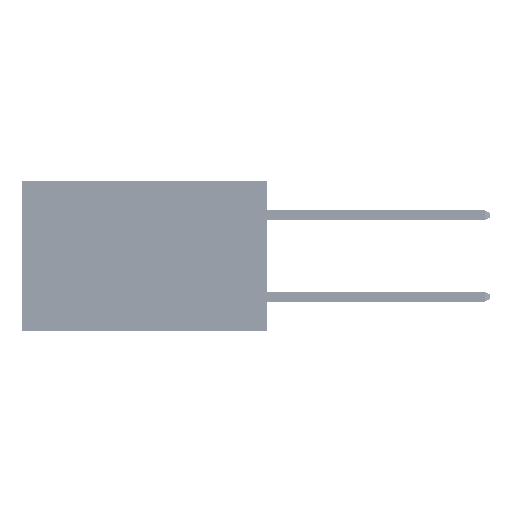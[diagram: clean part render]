
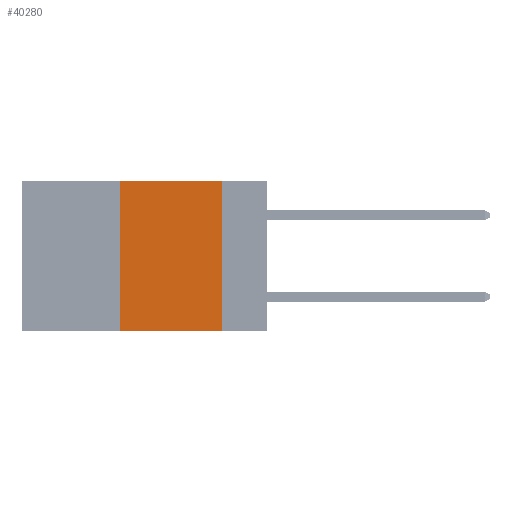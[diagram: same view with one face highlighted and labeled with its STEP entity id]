
A CAD part, left-side view. The second image highlights one B-rep face of the part: STEP entity #40280.
In plain terms, the highlighted planar face has unit normal (-1, 0, 0).
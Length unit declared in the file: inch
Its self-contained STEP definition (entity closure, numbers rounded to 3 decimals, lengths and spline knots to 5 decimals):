
#652 = EDGE_CURVE ( 'NONE', #5444, #50497, #5335, .T. ) ;
#2498 = CARTESIAN_POINT ( 'NONE',  ( 0., 0.11, 0. ) ) ;
#3532 = VECTOR ( 'NONE', #49097, 39.37008 ) ;
#4040 = CARTESIAN_POINT ( 'NONE',  ( 0., 0.36, 0. ) ) ;
#4802 = FACE_OUTER_BOUND ( 'NONE', #23849, .T. ) ;
#4806 = PLANE ( 'NONE',  #24379 ) ;
#5335 = LINE ( 'NONE', #4040, #3532 ) ;
#5444 = VERTEX_POINT ( 'NONE', #21013 ) ;
#6139 = DIRECTION ( 'NONE',  ( 0., -1., 0. ) ) ;
#6668 = LINE ( 'NONE', #2498, #26989 ) ;
#8266 = LINE ( 'NONE', #50133, #28001 ) ;
#8315 = EDGE_CURVE ( 'NONE', #50497, #37248, #40136, .T. ) ;
#9761 = ORIENTED_EDGE ( 'NONE', *, *, #8315, .F. ) ;
#9820 = ORIENTED_EDGE ( 'NONE', *, *, #652, .F. ) ;
#10383 = CARTESIAN_POINT ( 'NONE',  ( 0., 0.6, 0. ) ) ;
#13684 = DIRECTION ( 'NONE',  ( 0., 0., -1. ) ) ;
#18819 = DIRECTION ( 'NONE',  ( 0., 0., -1. ) ) ;
#21013 = CARTESIAN_POINT ( 'NONE',  ( 0., 0.36, -0.37 ) ) ;
#21772 = DIRECTION ( 'NONE',  ( 0., -1., 0. ) ) ;
#21999 = CARTESIAN_POINT ( 'NONE',  ( 0., 0.36, 0. ) ) ;
#23849 = EDGE_LOOP ( 'NONE', ( #24038, #9761, #9820, #44391 ) ) ;
#24038 = ORIENTED_EDGE ( 'NONE', *, *, #34368, .F. ) ;
#24379 = AXIS2_PLACEMENT_3D ( 'NONE', #42239, #50224, #13684 ) ;
#26989 = VECTOR ( 'NONE', #18819, 39.37008 ) ;
#28001 = VECTOR ( 'NONE', #6139, 39.37008 ) ;
#31786 = CARTESIAN_POINT ( 'NONE',  ( 0., 0.11, 0. ) ) ;
#34368 = EDGE_CURVE ( 'NONE', #37248, #34710, #6668, .T. ) ;
#34411 = VECTOR ( 'NONE', #21772, 39.37008 ) ;
#34710 = VERTEX_POINT ( 'NONE', #50078 ) ;
#37248 = VERTEX_POINT ( 'NONE', #31786 ) ;
#40136 = LINE ( 'NONE', #10383, #34411 ) ;
#40280 = ADVANCED_FACE ( 'NONE', ( #4802 ), #4806, .F. ) ;
#42239 = CARTESIAN_POINT ( 'NONE',  ( 0., 0.6, 0. ) ) ;
#43167 = EDGE_CURVE ( 'NONE', #5444, #34710, #8266, .T. ) ;
#44391 = ORIENTED_EDGE ( 'NONE', *, *, #43167, .T. ) ;
#49097 = DIRECTION ( 'NONE',  ( 0., 0., 1. ) ) ;
#50078 = CARTESIAN_POINT ( 'NONE',  ( 0., 0.11, -0.37 ) ) ;
#50133 = CARTESIAN_POINT ( 'NONE',  ( 0., 0.6, -0.37 ) ) ;
#50224 = DIRECTION ( 'NONE',  ( 1., 0., 0. ) ) ;
#50497 = VERTEX_POINT ( 'NONE', #21999 ) ;
